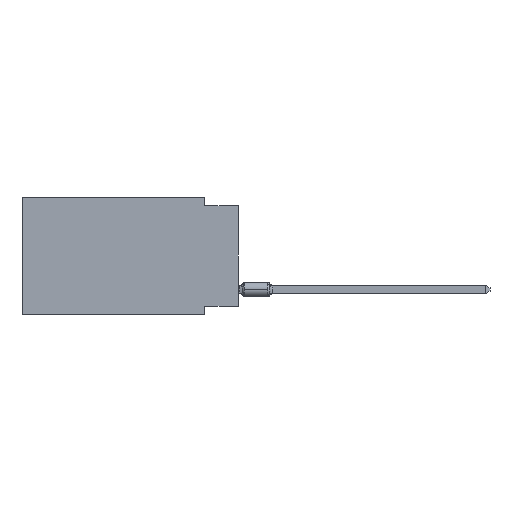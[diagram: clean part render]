
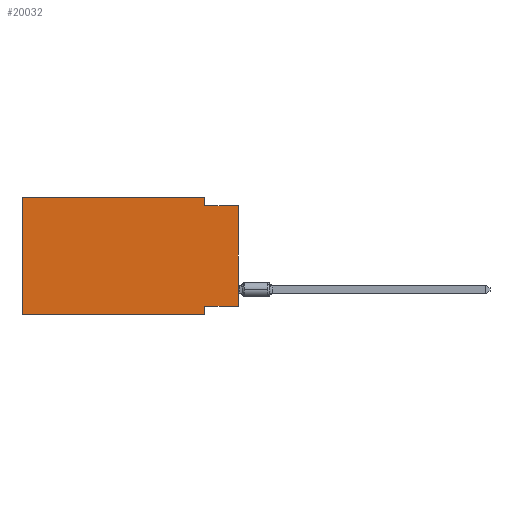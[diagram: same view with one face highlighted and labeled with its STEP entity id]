
A CAD part, left-side view. The second image highlights one B-rep face of the part: STEP entity #20032.
In plain terms, the highlighted planar face has unit normal (-1, 0, 0).
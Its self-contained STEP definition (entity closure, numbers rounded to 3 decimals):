
#37 = VERTEX_POINT ( 'NONE', #33619 ) ;
#250 = VERTEX_POINT ( 'NONE', #26490 ) ;
#275 = CARTESIAN_POINT ( 'NONE',  ( 0., 2.54, -8.255 ) ) ;
#382 = CARTESIAN_POINT ( 'NONE',  ( 0., 16.383, 0. ) ) ;
#629 = ORIENTED_EDGE ( 'NONE', *, *, #34254, .F. ) ;
#1078 = CARTESIAN_POINT ( 'NONE',  ( 0., 0., 0. ) ) ;
#2372 = ORIENTED_EDGE ( 'NONE', *, *, #12767, .F. ) ;
#2924 = PLANE ( 'NONE',  #3496 ) ;
#3339 = VECTOR ( 'NONE', #15962, 1000. ) ;
#3496 = AXIS2_PLACEMENT_3D ( 'NONE', #382, #5843, #11875 ) ;
#4160 = DIRECTION ( 'NONE',  ( 0., 0., 1. ) ) ;
#5352 = VERTEX_POINT ( 'NONE', #9508 ) ;
#5843 = DIRECTION ( 'NONE',  ( 1., 0., 0. ) ) ;
#6114 = EDGE_CURVE ( 'NONE', #24593, #7082, #13249, .T. ) ;
#6621 = ORIENTED_EDGE ( 'NONE', *, *, #28031, .T. ) ;
#7082 = VERTEX_POINT ( 'NONE', #16763 ) ;
#7945 = CARTESIAN_POINT ( 'NONE',  ( 0., 16.383, 0. ) ) ;
#8217 = CARTESIAN_POINT ( 'NONE',  ( 0., 0., -8.255 ) ) ;
#8333 = CARTESIAN_POINT ( 'NONE',  ( 0., 2.54, -8.89 ) ) ;
#9497 = DIRECTION ( 'NONE',  ( 0., 1., 0. ) ) ;
#9508 = CARTESIAN_POINT ( 'NONE',  ( 0., 16.383, 0. ) ) ;
#9847 = LINE ( 'NONE', #12951, #28783 ) ;
#10154 = CARTESIAN_POINT ( 'NONE',  ( 0., 16.383, -8.89 ) ) ;
#11135 = ORIENTED_EDGE ( 'NONE', *, *, #28342, .F. ) ;
#11231 = VECTOR ( 'NONE', #17105, 1000. ) ;
#11370 = VERTEX_POINT ( 'NONE', #31032 ) ;
#11462 = LINE ( 'NONE', #20045, #21645 ) ;
#11741 = ORIENTED_EDGE ( 'NONE', *, *, #6114, .T. ) ;
#11875 = DIRECTION ( 'NONE',  ( 0., 0., -1. ) ) ;
#12404 = ORIENTED_EDGE ( 'NONE', *, *, #24495, .F. ) ;
#12459 = ORIENTED_EDGE ( 'NONE', *, *, #34560, .F. ) ;
#12767 = EDGE_CURVE ( 'NONE', #30512, #28697, #23363, .T. ) ;
#12951 = CARTESIAN_POINT ( 'NONE',  ( 0., 0., -0.635 ) ) ;
#13249 = LINE ( 'NONE', #10154, #17177 ) ;
#15962 = DIRECTION ( 'NONE',  ( 0., 0., -1. ) ) ;
#16763 = CARTESIAN_POINT ( 'NONE',  ( 0., 2.54, -8.89 ) ) ;
#17105 = DIRECTION ( 'NONE',  ( 0., 0., -1. ) ) ;
#17177 = VECTOR ( 'NONE', #24197, 1000. ) ;
#17648 = VECTOR ( 'NONE', #4160, 1000. ) ;
#17931 = VECTOR ( 'NONE', #25237, 1000. ) ;
#19269 = VECTOR ( 'NONE', #9497, 1000. ) ;
#20032 = ADVANCED_FACE ( 'NONE', ( #22820 ), #2924, .F. ) ;
#20045 = CARTESIAN_POINT ( 'NONE',  ( 0., 16.383, 0. ) ) ;
#20092 = EDGE_LOOP ( 'NONE', ( #6621, #12404, #28209, #629, #12459, #11741, #11135, #2372 ) ) ;
#21422 = LINE ( 'NONE', #29618, #3339 ) ;
#21513 = CARTESIAN_POINT ( 'NONE',  ( 0., 16.383, -8.89 ) ) ;
#21645 = VECTOR ( 'NONE', #22581, 1000. ) ;
#22581 = DIRECTION ( 'NONE',  ( 0., -1., 0. ) ) ;
#22820 = FACE_OUTER_BOUND ( 'NONE', #20092, .T. ) ;
#23363 = LINE ( 'NONE', #34472, #19269 ) ;
#23646 = EDGE_CURVE ( 'NONE', #250, #11370, #21422, .T. ) ;
#24197 = DIRECTION ( 'NONE',  ( 0., -1., 0. ) ) ;
#24495 = EDGE_CURVE ( 'NONE', #11370, #37, #9847, .T. ) ;
#24593 = VERTEX_POINT ( 'NONE', #21513 ) ;
#25237 = DIRECTION ( 'NONE',  ( 0., 0., 1. ) ) ;
#26067 = LINE ( 'NONE', #1078, #17648 ) ;
#26490 = CARTESIAN_POINT ( 'NONE',  ( 0., 2.54, 0. ) ) ;
#27844 = LINE ( 'NONE', #8333, #11231 ) ;
#27961 = LINE ( 'NONE', #7945, #17931 ) ;
#28031 = EDGE_CURVE ( 'NONE', #30512, #37, #26067, .T. ) ;
#28209 = ORIENTED_EDGE ( 'NONE', *, *, #23646, .F. ) ;
#28342 = EDGE_CURVE ( 'NONE', #28697, #7082, #27844, .T. ) ;
#28697 = VERTEX_POINT ( 'NONE', #275 ) ;
#28783 = VECTOR ( 'NONE', #34650, 1000. ) ;
#29618 = CARTESIAN_POINT ( 'NONE',  ( 0., 2.54, 0. ) ) ;
#30512 = VERTEX_POINT ( 'NONE', #8217 ) ;
#31032 = CARTESIAN_POINT ( 'NONE',  ( 0., 2.54, -0.635 ) ) ;
#33619 = CARTESIAN_POINT ( 'NONE',  ( 0., 0., -0.635 ) ) ;
#34254 = EDGE_CURVE ( 'NONE', #5352, #250, #11462, .T. ) ;
#34472 = CARTESIAN_POINT ( 'NONE',  ( 0., 0., -8.255 ) ) ;
#34560 = EDGE_CURVE ( 'NONE', #24593, #5352, #27961, .T. ) ;
#34650 = DIRECTION ( 'NONE',  ( 0., -1., 0. ) ) ;
